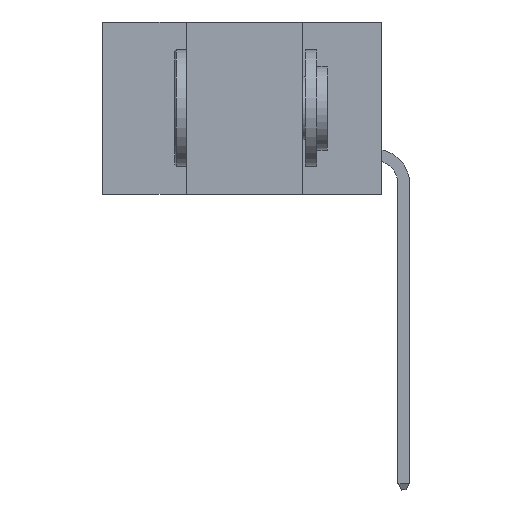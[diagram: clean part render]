
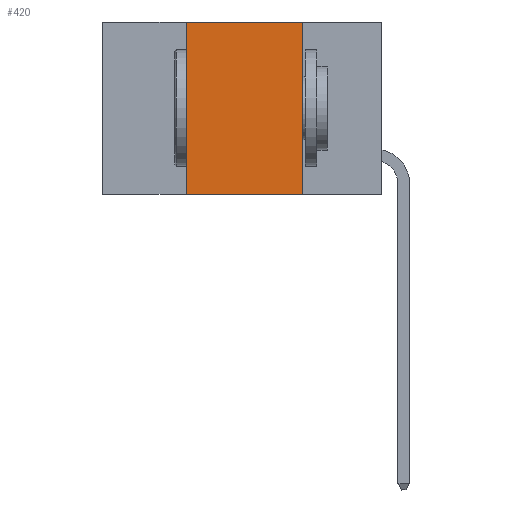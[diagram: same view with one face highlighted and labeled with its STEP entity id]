
A CAD part, left-side view. The second image highlights one B-rep face of the part: STEP entity #420.
In plain terms, the highlighted planar face has unit normal (-1, 0, 0).
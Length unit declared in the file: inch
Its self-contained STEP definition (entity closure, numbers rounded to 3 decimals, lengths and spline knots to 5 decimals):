
#285 = ORIENTED_EDGE ( 'NONE', *, *, #7376, .F. ) ;
#420 = ADVANCED_FACE ( 'NONE', ( #16020 ), #11175, .F. ) ;
#741 = DIRECTION ( 'NONE',  ( 0., -1., 0. ) ) ;
#809 = EDGE_LOOP ( 'NONE', ( #11422, #16206, #285, #8614 ) ) ;
#1151 = CARTESIAN_POINT ( 'NONE',  ( 0., 0.42, -0.37 ) ) ;
#1993 = EDGE_CURVE ( 'NONE', #14816, #15548, #14112, .T. ) ;
#2120 = VECTOR ( 'NONE', #16033, 39.37008 ) ;
#2409 = CARTESIAN_POINT ( 'NONE',  ( 0., 0.42, 0. ) ) ;
#2426 = EDGE_CURVE ( 'NONE', #4003, #4932, #16139, .T. ) ;
#4003 = VERTEX_POINT ( 'NONE', #1151 ) ;
#4158 = CARTESIAN_POINT ( 'NONE',  ( 0., 0.6, -0.37 ) ) ;
#4932 = VERTEX_POINT ( 'NONE', #11763 ) ;
#5747 = VECTOR ( 'NONE', #6208, 39.37008 ) ;
#6012 = CARTESIAN_POINT ( 'NONE',  ( 0., 0.6, 0. ) ) ;
#6208 = DIRECTION ( 'NONE',  ( 0., 0., 1. ) ) ;
#7297 = CARTESIAN_POINT ( 'NONE',  ( 0., 0.17, 0. ) ) ;
#7376 = EDGE_CURVE ( 'NONE', #4003, #14816, #11544, .T. ) ;
#7426 = DIRECTION ( 'NONE',  ( 0., 0., -1. ) ) ;
#7986 = LINE ( 'NONE', #15104, #10698 ) ;
#8146 = AXIS2_PLACEMENT_3D ( 'NONE', #15135, #16590, #16422 ) ;
#8349 = EDGE_CURVE ( 'NONE', #15548, #4932, #7986, .T. ) ;
#8614 = ORIENTED_EDGE ( 'NONE', *, *, #2426, .T. ) ;
#8727 = VECTOR ( 'NONE', #741, 39.37008 ) ;
#9376 = CARTESIAN_POINT ( 'NONE',  ( 0., 0.42, 0. ) ) ;
#10698 = VECTOR ( 'NONE', #7426, 39.37008 ) ;
#11175 = PLANE ( 'NONE',  #8146 ) ;
#11422 = ORIENTED_EDGE ( 'NONE', *, *, #8349, .F. ) ;
#11544 = LINE ( 'NONE', #2409, #5747 ) ;
#11763 = CARTESIAN_POINT ( 'NONE',  ( 0., 0.17, -0.37 ) ) ;
#14112 = LINE ( 'NONE', #6012, #8727 ) ;
#14816 = VERTEX_POINT ( 'NONE', #9376 ) ;
#15104 = CARTESIAN_POINT ( 'NONE',  ( 0., 0.17, 0. ) ) ;
#15135 = CARTESIAN_POINT ( 'NONE',  ( 0., 0.6, 0. ) ) ;
#15548 = VERTEX_POINT ( 'NONE', #7297 ) ;
#16020 = FACE_OUTER_BOUND ( 'NONE', #809, .T. ) ;
#16033 = DIRECTION ( 'NONE',  ( 0., -1., 0. ) ) ;
#16139 = LINE ( 'NONE', #4158, #2120 ) ;
#16206 = ORIENTED_EDGE ( 'NONE', *, *, #1993, .F. ) ;
#16422 = DIRECTION ( 'NONE',  ( 0., 0., -1. ) ) ;
#16590 = DIRECTION ( 'NONE',  ( 1., 0., 0. ) ) ;
